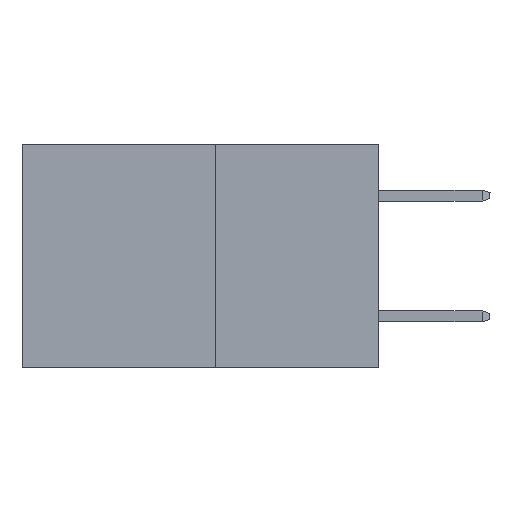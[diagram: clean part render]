
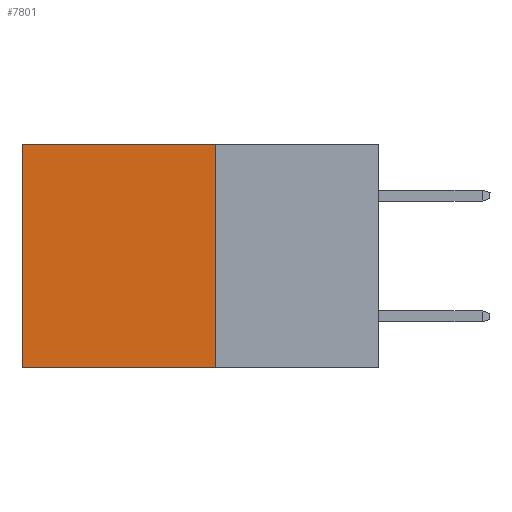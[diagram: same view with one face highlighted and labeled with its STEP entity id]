
A CAD part, left-side view. The second image highlights one B-rep face of the part: STEP entity #7801.
In plain terms, the highlighted planar face has unit normal (-1, 0, 0).
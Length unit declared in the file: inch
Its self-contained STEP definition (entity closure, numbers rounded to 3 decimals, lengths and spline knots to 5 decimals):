
#341 = EDGE_LOOP ( 'NONE', ( #9733, #17384, #17270, #12444 ) ) ;
#818 = LINE ( 'NONE', #1381, #14299 ) ;
#968 = VERTEX_POINT ( 'NONE', #5066 ) ;
#1093 = DIRECTION ( 'NONE',  ( 0., 0., -1. ) ) ;
#1381 = CARTESIAN_POINT ( 'NONE',  ( 0.277, 0.27, -0.37 ) ) ;
#1689 = EDGE_CURVE ( 'NONE', #14979, #17875, #4464, .T. ) ;
#2822 = EDGE_CURVE ( 'NONE', #20353, #17875, #4673, .T. ) ;
#3065 = DIRECTION ( 'NONE',  ( 0., 1., 0. ) ) ;
#3262 = CARTESIAN_POINT ( 'NONE',  ( 0.277, 0.27, -0.37 ) ) ;
#4464 = LINE ( 'NONE', #8643, #20439 ) ;
#4483 = CARTESIAN_POINT ( 'NONE',  ( 0.277, 0.27, -0.37 ) ) ;
#4673 = LINE ( 'NONE', #3262, #13033 ) ;
#5066 = CARTESIAN_POINT ( 'NONE',  ( 0.277, 0.27, 0. ) ) ;
#6964 = EDGE_CURVE ( 'NONE', #968, #20353, #818, .T. ) ;
#7801 = ADVANCED_FACE ( 'NONE', ( #15276 ), #10511, .F. ) ;
#8643 = CARTESIAN_POINT ( 'NONE',  ( 0.277, 0.59, -0.37 ) ) ;
#9361 = CARTESIAN_POINT ( 'NONE',  ( 0.277, 0.59, -0.37 ) ) ;
#9733 = ORIENTED_EDGE ( 'NONE', *, *, #1689, .T. ) ;
#10278 = CARTESIAN_POINT ( 'NONE',  ( 0.277, 0.27, 0. ) ) ;
#10455 = DIRECTION ( 'NONE',  ( 0., 0., -1. ) ) ;
#10462 = DIRECTION ( 'NONE',  ( 1., 0., 0. ) ) ;
#10511 = PLANE ( 'NONE',  #11305 ) ;
#10662 = CARTESIAN_POINT ( 'NONE',  ( 0.277, 0.27, -0.37 ) ) ;
#11305 = AXIS2_PLACEMENT_3D ( 'NONE', #10662, #10462, #10455 ) ;
#12444 = ORIENTED_EDGE ( 'NONE', *, *, #16910, .T. ) ;
#13033 = VECTOR ( 'NONE', #3065, 39.37008 ) ;
#14299 = VECTOR ( 'NONE', #1093, 39.37008 ) ;
#14979 = VERTEX_POINT ( 'NONE', #18253 ) ;
#15257 = DIRECTION ( 'NONE',  ( 0., 1., 0. ) ) ;
#15276 = FACE_OUTER_BOUND ( 'NONE', #341, .T. ) ;
#16910 = EDGE_CURVE ( 'NONE', #968, #14979, #19056, .T. ) ;
#17270 = ORIENTED_EDGE ( 'NONE', *, *, #6964, .F. ) ;
#17384 = ORIENTED_EDGE ( 'NONE', *, *, #2822, .F. ) ;
#17875 = VERTEX_POINT ( 'NONE', #9361 ) ;
#18253 = CARTESIAN_POINT ( 'NONE',  ( 0.277, 0.59, 0. ) ) ;
#18544 = VECTOR ( 'NONE', #15257, 39.37008 ) ;
#19056 = LINE ( 'NONE', #10278, #18544 ) ;
#20353 = VERTEX_POINT ( 'NONE', #4483 ) ;
#20439 = VECTOR ( 'NONE', #21058, 39.37008 ) ;
#21058 = DIRECTION ( 'NONE',  ( 0., 0., -1. ) ) ;
